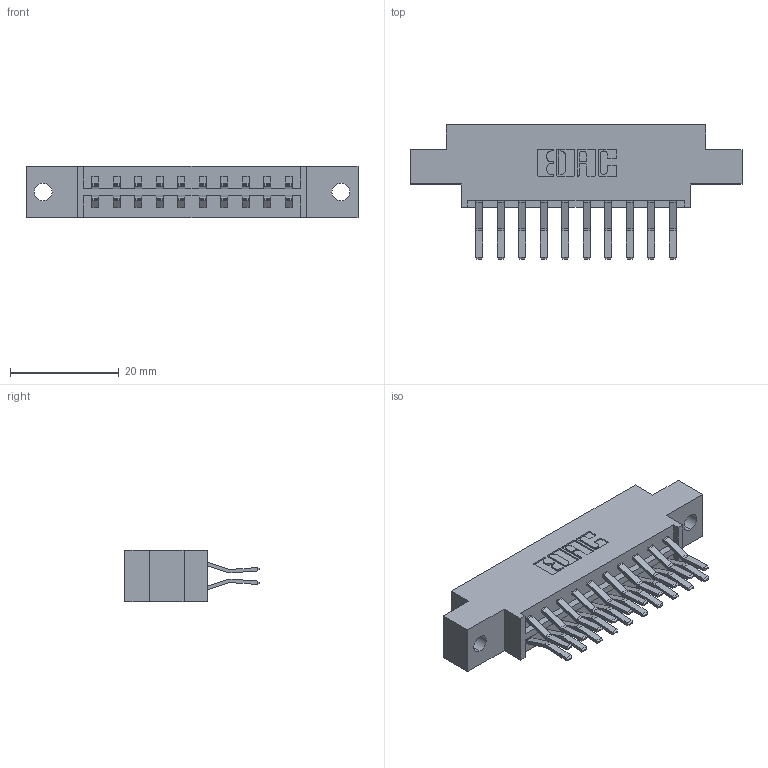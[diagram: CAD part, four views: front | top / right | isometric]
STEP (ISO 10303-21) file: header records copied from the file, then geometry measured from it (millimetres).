
FILE_DESCRIPTION (( 'STEP AP203' ), '1' );
FILE_NAME ('833-020-560-802.STEP', '2020-06-01T14:21:55', ( '' ), ( '' ), 'SwSTEP 2.0', 'SolidWorks 2020', '' );
FILE_SCHEMA (( 'CONFIG_CONTROL_DESIGN' ));
Length unit declared in the file: inch
Products named in the file (3): 345-292-001_560 Tail; 833 Part_Offset - .128 Dia; 833-020-560-802
Assembly tree (21 placements, depth 2):
  833-020-560-802
    833 Part_Offset - .128 Dia
    345-292-001_560 Tail  x20
Bounding box: 61.16 x 24.78 x 9.4 mm (x, y, z)
Volume: 5811.8 mm3; surface area: 6848.6 mm2
Topology: 21 solids, 21 shells, 1198 faces, 3543 edges, 2334 vertices
Faces by surface type: plane 794, cylinder 404
Entity records: 10795 total; most frequent: CARTESIAN_POINT 1830, ORIENTED_EDGE 1766, DIRECTION 1623, EDGE_CURVE 883, LINE 751, VECTOR 751, VERTEX_POINT 586, AXIS2_PLACEMENT_3D 436
